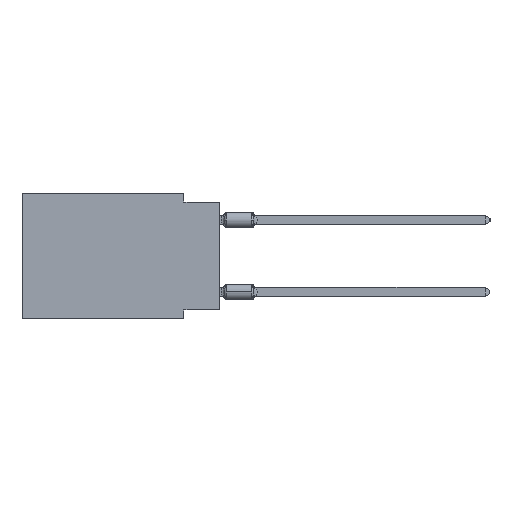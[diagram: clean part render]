
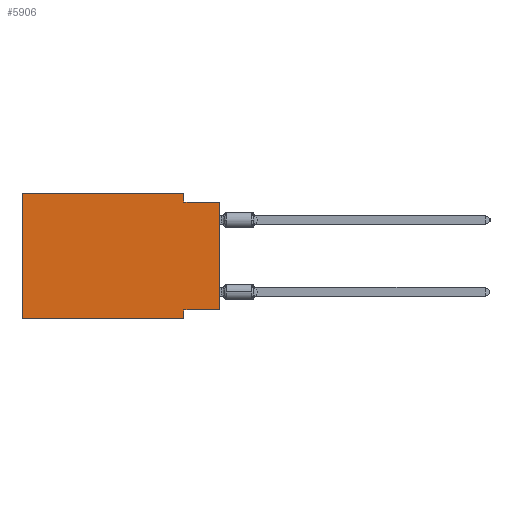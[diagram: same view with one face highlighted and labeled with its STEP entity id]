
A CAD part, left-side view. The second image highlights one B-rep face of the part: STEP entity #5906.
In plain terms, the highlighted planar face has unit normal (-1, 0, 0).
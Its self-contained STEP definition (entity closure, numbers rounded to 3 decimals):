
#89 = DIRECTION ( 'NONE',  ( 0., 0., 1. ) ) ;
#556 = ORIENTED_EDGE ( 'NONE', *, *, #5590, .F. ) ;
#560 = CARTESIAN_POINT ( 'NONE',  ( 0., 2.54, 0. ) ) ;
#888 = ORIENTED_EDGE ( 'NONE', *, *, #25335, .F. ) ;
#1255 = CARTESIAN_POINT ( 'NONE',  ( 0., 13.97, -8.89 ) ) ;
#2014 = FACE_OUTER_BOUND ( 'NONE', #15419, .T. ) ;
#3240 = DIRECTION ( 'NONE',  ( 0., 0., -1. ) ) ;
#3882 = VERTEX_POINT ( 'NONE', #30738 ) ;
#5590 = EDGE_CURVE ( 'NONE', #18464, #3882, #30982, .T. ) ;
#5735 = ORIENTED_EDGE ( 'NONE', *, *, #30952, .T. ) ;
#5906 = ADVANCED_FACE ( 'NONE', ( #2014 ), #39191, .F. ) ;
#6473 = VERTEX_POINT ( 'NONE', #39530 ) ;
#8109 = ORIENTED_EDGE ( 'NONE', *, *, #35214, .F. ) ;
#9554 = VECTOR ( 'NONE', #37382, 1000. ) ;
#9862 = CARTESIAN_POINT ( 'NONE',  ( 0., 2.54, -8.89 ) ) ;
#10807 = LINE ( 'NONE', #38718, #34572 ) ;
#11805 = VERTEX_POINT ( 'NONE', #23257 ) ;
#12193 = CARTESIAN_POINT ( 'NONE',  ( 0., 2.54, -8.89 ) ) ;
#12405 = VERTEX_POINT ( 'NONE', #34762 ) ;
#14302 = ORIENTED_EDGE ( 'NONE', *, *, #39465, .F. ) ;
#14308 = VECTOR ( 'NONE', #89, 1000. ) ;
#15419 = EDGE_LOOP ( 'NONE', ( #5735, #27784, #556, #26435, #8109, #19929, #14302, #888 ) ) ;
#16331 = EDGE_CURVE ( 'NONE', #3882, #11805, #18234, .T. ) ;
#17247 = DIRECTION ( 'NONE',  ( 0., -1., 0. ) ) ;
#18234 = LINE ( 'NONE', #33306, #33821 ) ;
#18464 = VERTEX_POINT ( 'NONE', #560 ) ;
#18905 = CARTESIAN_POINT ( 'NONE',  ( 0., 13.97, 0. ) ) ;
#19145 = AXIS2_PLACEMENT_3D ( 'NONE', #33150, #23731, #36178 ) ;
#19929 = ORIENTED_EDGE ( 'NONE', *, *, #26684, .T. ) ;
#20665 = DIRECTION ( 'NONE',  ( 0., -1., 0. ) ) ;
#23257 = CARTESIAN_POINT ( 'NONE',  ( 0., 0., -0.635 ) ) ;
#23731 = DIRECTION ( 'NONE',  ( 1., 0., 0. ) ) ;
#23848 = CARTESIAN_POINT ( 'NONE',  ( 0., 0., 0. ) ) ;
#24439 = LINE ( 'NONE', #12193, #36940 ) ;
#25335 = EDGE_CURVE ( 'NONE', #12405, #6473, #10807, .T. ) ;
#25870 = DIRECTION ( 'NONE',  ( 0., 1., 0. ) ) ;
#26083 = CARTESIAN_POINT ( 'NONE',  ( 0., 13.97, -8.89 ) ) ;
#26276 = DIRECTION ( 'NONE',  ( 0., -1., 0. ) ) ;
#26435 = ORIENTED_EDGE ( 'NONE', *, *, #31973, .F. ) ;
#26484 = LINE ( 'NONE', #26083, #28868 ) ;
#26668 = LINE ( 'NONE', #38911, #31652 ) ;
#26684 = EDGE_CURVE ( 'NONE', #28607, #36462, #26484, .T. ) ;
#27775 = CARTESIAN_POINT ( 'NONE',  ( 0., 2.54, 0. ) ) ;
#27784 = ORIENTED_EDGE ( 'NONE', *, *, #16331, .F. ) ;
#28607 = VERTEX_POINT ( 'NONE', #1255 ) ;
#28868 = VECTOR ( 'NONE', #17247, 1000. ) ;
#30738 = CARTESIAN_POINT ( 'NONE',  ( 0., 2.54, -0.635 ) ) ;
#30952 = EDGE_CURVE ( 'NONE', #12405, #11805, #39496, .T. ) ;
#30982 = LINE ( 'NONE', #27775, #38975 ) ;
#31652 = VECTOR ( 'NONE', #26276, 1000. ) ;
#31973 = EDGE_CURVE ( 'NONE', #36670, #18464, #26668, .T. ) ;
#33150 = CARTESIAN_POINT ( 'NONE',  ( 0., 13.97, 0. ) ) ;
#33306 = CARTESIAN_POINT ( 'NONE',  ( 0., 0., -0.635 ) ) ;
#33672 = DIRECTION ( 'NONE',  ( 0., 0., -1. ) ) ;
#33821 = VECTOR ( 'NONE', #20665, 1000. ) ;
#34572 = VECTOR ( 'NONE', #25870, 1000. ) ;
#34762 = CARTESIAN_POINT ( 'NONE',  ( 0., 0., -8.255 ) ) ;
#35214 = EDGE_CURVE ( 'NONE', #28607, #36670, #36595, .T. ) ;
#36178 = DIRECTION ( 'NONE',  ( 0., 0., -1. ) ) ;
#36462 = VERTEX_POINT ( 'NONE', #9862 ) ;
#36595 = LINE ( 'NONE', #18905, #9554 ) ;
#36670 = VERTEX_POINT ( 'NONE', #38371 ) ;
#36940 = VECTOR ( 'NONE', #33672, 1000. ) ;
#37382 = DIRECTION ( 'NONE',  ( 0., 0., 1. ) ) ;
#38371 = CARTESIAN_POINT ( 'NONE',  ( 0., 13.97, 0. ) ) ;
#38718 = CARTESIAN_POINT ( 'NONE',  ( 0., 0., -8.255 ) ) ;
#38911 = CARTESIAN_POINT ( 'NONE',  ( 0., 13.97, 0. ) ) ;
#38975 = VECTOR ( 'NONE', #3240, 1000. ) ;
#39191 = PLANE ( 'NONE',  #19145 ) ;
#39465 = EDGE_CURVE ( 'NONE', #6473, #36462, #24439, .T. ) ;
#39496 = LINE ( 'NONE', #23848, #14308 ) ;
#39530 = CARTESIAN_POINT ( 'NONE',  ( 0., 2.54, -8.255 ) ) ;
